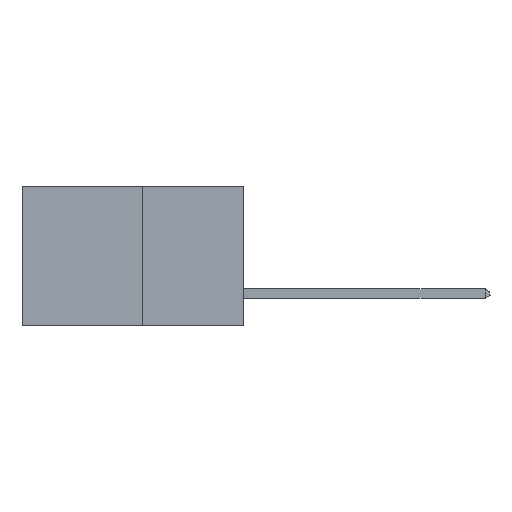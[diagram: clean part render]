
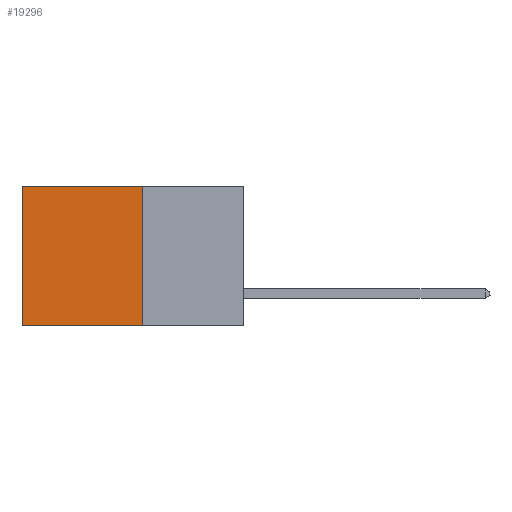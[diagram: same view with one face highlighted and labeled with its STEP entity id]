
A CAD part, left-side view. The second image highlights one B-rep face of the part: STEP entity #19296.
In plain terms, the highlighted planar face has unit normal (-1, 0, 0).
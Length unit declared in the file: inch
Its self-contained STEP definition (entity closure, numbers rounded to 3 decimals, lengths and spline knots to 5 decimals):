
#396 = DIRECTION ( 'NONE',  ( 0., 1., 0. ) ) ;
#1698 = DIRECTION ( 'NONE',  ( 0., 0., -1. ) ) ;
#2153 = CARTESIAN_POINT ( 'NONE',  ( 0.277, 0.27, -0.37 ) ) ;
#2538 = VECTOR ( 'NONE', #6098, 39.37008 ) ;
#2990 = VECTOR ( 'NONE', #396, 39.37008 ) ;
#3788 = FACE_OUTER_BOUND ( 'NONE', #7030, .T. ) ;
#3933 = DIRECTION ( 'NONE',  ( 1., 0., 0. ) ) ;
#3959 = VERTEX_POINT ( 'NONE', #2153 ) ;
#6098 = DIRECTION ( 'NONE',  ( 0., 0., -1. ) ) ;
#7030 = EDGE_LOOP ( 'NONE', ( #15221, #9795, #23439, #22197 ) ) ;
#7122 = AXIS2_PLACEMENT_3D ( 'NONE', #26857, #3933, #1698 ) ;
#8240 = CARTESIAN_POINT ( 'NONE',  ( 0.277, 0.59, -0.37 ) ) ;
#8375 = VERTEX_POINT ( 'NONE', #25411 ) ;
#9139 = EDGE_CURVE ( 'NONE', #23385, #28178, #25684, .T. ) ;
#9795 = ORIENTED_EDGE ( 'NONE', *, *, #25435, .F. ) ;
#10595 = VECTOR ( 'NONE', #28765, 39.37008 ) ;
#11583 = DIRECTION ( 'NONE',  ( 0., 1., 0. ) ) ;
#11667 = CARTESIAN_POINT ( 'NONE',  ( 0.277, 0.27, 0. ) ) ;
#12868 = CARTESIAN_POINT ( 'NONE',  ( 0.277, 0.59, 0. ) ) ;
#14574 = LINE ( 'NONE', #27856, #2990 ) ;
#15221 = ORIENTED_EDGE ( 'NONE', *, *, #28176, .T. ) ;
#17489 = LINE ( 'NONE', #8240, #10595 ) ;
#19296 = ADVANCED_FACE ( 'NONE', ( #3788 ), #29092, .F. ) ;
#19908 = CARTESIAN_POINT ( 'NONE',  ( 0.277, 0.27, -0.37 ) ) ;
#20522 = EDGE_CURVE ( 'NONE', #23385, #3959, #26228, .T. ) ;
#22197 = ORIENTED_EDGE ( 'NONE', *, *, #9139, .T. ) ;
#23385 = VERTEX_POINT ( 'NONE', #26985 ) ;
#23439 = ORIENTED_EDGE ( 'NONE', *, *, #20522, .F. ) ;
#24985 = VECTOR ( 'NONE', #11583, 39.37008 ) ;
#25411 = CARTESIAN_POINT ( 'NONE',  ( 0.277, 0.59, -0.37 ) ) ;
#25435 = EDGE_CURVE ( 'NONE', #3959, #8375, #14574, .T. ) ;
#25684 = LINE ( 'NONE', #11667, #24985 ) ;
#26228 = LINE ( 'NONE', #19908, #2538 ) ;
#26857 = CARTESIAN_POINT ( 'NONE',  ( 0.277, 0.27, -0.37 ) ) ;
#26985 = CARTESIAN_POINT ( 'NONE',  ( 0.277, 0.27, 0. ) ) ;
#27856 = CARTESIAN_POINT ( 'NONE',  ( 0.277, 0.27, -0.37 ) ) ;
#28176 = EDGE_CURVE ( 'NONE', #28178, #8375, #17489, .T. ) ;
#28178 = VERTEX_POINT ( 'NONE', #12868 ) ;
#28765 = DIRECTION ( 'NONE',  ( 0., 0., -1. ) ) ;
#29092 = PLANE ( 'NONE',  #7122 ) ;
